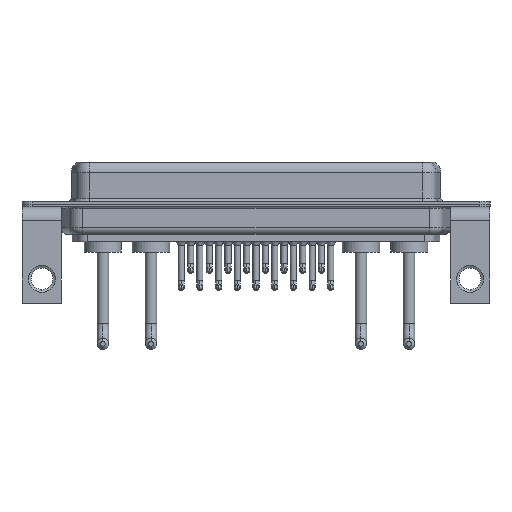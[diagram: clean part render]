
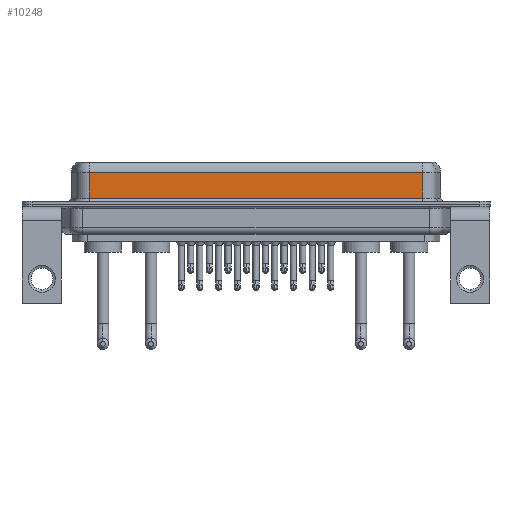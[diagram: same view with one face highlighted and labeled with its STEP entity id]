
A CAD part, front view. The second image highlights one B-rep face of the part: STEP entity #10248.
In plain terms, the highlighted planar face has unit normal (0, -1, 0).
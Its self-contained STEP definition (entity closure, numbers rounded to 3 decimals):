
#250 = LINE ( 'NONE', #8896, #5205 ) ;
#1633 = VERTEX_POINT ( 'NONE', #10551 ) ;
#2014 = EDGE_LOOP ( 'NONE', ( #5962, #17339, #8082, #9317 ) ) ;
#2070 = LINE ( 'NONE', #7122, #5379 ) ;
#3595 = DIRECTION ( 'NONE',  ( 0., 1., 0. ) ) ;
#3882 = CARTESIAN_POINT ( 'NONE',  ( 7.038, -3.95, 4.65 ) ) ;
#4285 = AXIS2_PLACEMENT_3D ( 'NONE', #10390, #3595, #6930 ) ;
#5146 = CARTESIAN_POINT ( 'NONE',  ( 56.462, -3.95, 4.65 ) ) ;
#5170 = CARTESIAN_POINT ( 'NONE',  ( 56.462, -3.95, 0.9 ) ) ;
#5205 = VECTOR ( 'NONE', #20997, 1000. ) ;
#5209 = PLANE ( 'NONE',  #4285 ) ;
#5379 = VECTOR ( 'NONE', #7241, 1000. ) ;
#5962 = ORIENTED_EDGE ( 'NONE', *, *, #8821, .F. ) ;
#6863 = VERTEX_POINT ( 'NONE', #5170 ) ;
#6930 = DIRECTION ( 'NONE',  ( 0., 0., 1. ) ) ;
#7122 = CARTESIAN_POINT ( 'NONE',  ( 56.462, -3.95, 6.4 ) ) ;
#7241 = DIRECTION ( 'NONE',  ( 0., 0., -1. ) ) ;
#7628 = CARTESIAN_POINT ( 'NONE',  ( 56.462, -3.95, 4.65 ) ) ;
#8082 = ORIENTED_EDGE ( 'NONE', *, *, #15701, .T. ) ;
#8666 = VECTOR ( 'NONE', #21703, 1000. ) ;
#8821 = EDGE_CURVE ( 'NONE', #12479, #6863, #2070, .T. ) ;
#8896 = CARTESIAN_POINT ( 'NONE',  ( 7.038, -3.95, 6.4 ) ) ;
#9317 = ORIENTED_EDGE ( 'NONE', *, *, #16458, .T. ) ;
#10248 = ADVANCED_FACE ( 'NONE', ( #19054 ), #5209, .F. ) ;
#10390 = CARTESIAN_POINT ( 'NONE',  ( 56.462, -3.95, 6.4 ) ) ;
#10551 = CARTESIAN_POINT ( 'NONE',  ( 7.038, -3.95, 0.9 ) ) ;
#10818 = VECTOR ( 'NONE', #17358, 1000. ) ;
#12479 = VERTEX_POINT ( 'NONE', #5146 ) ;
#13745 = VERTEX_POINT ( 'NONE', #3882 ) ;
#15610 = LINE ( 'NONE', #18736, #10818 ) ;
#15701 = EDGE_CURVE ( 'NONE', #13745, #1633, #250, .T. ) ;
#16286 = LINE ( 'NONE', #7628, #8666 ) ;
#16458 = EDGE_CURVE ( 'NONE', #1633, #6863, #15610, .T. ) ;
#17339 = ORIENTED_EDGE ( 'NONE', *, *, #17918, .T. ) ;
#17358 = DIRECTION ( 'NONE',  ( 1., 0., 0. ) ) ;
#17918 = EDGE_CURVE ( 'NONE', #12479, #13745, #16286, .T. ) ;
#18736 = CARTESIAN_POINT ( 'NONE',  ( 56.462, -3.95, 0.9 ) ) ;
#19054 = FACE_OUTER_BOUND ( 'NONE', #2014, .T. ) ;
#20997 = DIRECTION ( 'NONE',  ( 0., 0., -1. ) ) ;
#21703 = DIRECTION ( 'NONE',  ( -1., 0., 0. ) ) ;
